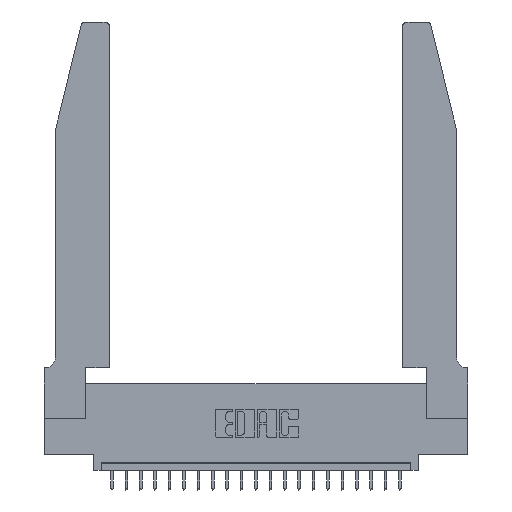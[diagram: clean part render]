
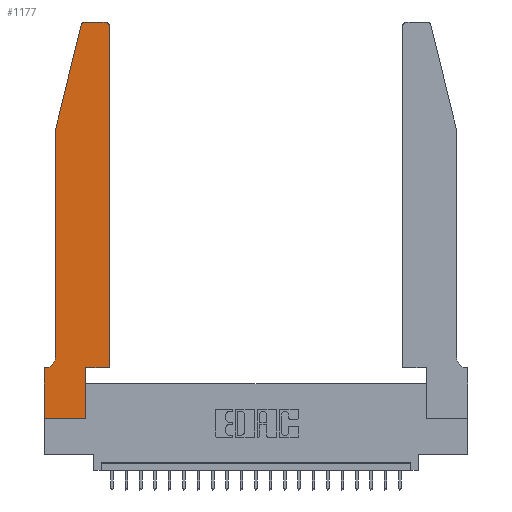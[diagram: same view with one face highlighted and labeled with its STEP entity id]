
A CAD part, top view. The second image highlights one B-rep face of the part: STEP entity #1177.
In plain terms, the highlighted planar face has unit normal (0, 0, 1).
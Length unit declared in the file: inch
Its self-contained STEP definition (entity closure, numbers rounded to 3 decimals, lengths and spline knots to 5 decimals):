
#88 = EDGE_CURVE ( 'NONE', #14024, #15743, #11137, .T. ) ;
#162 = EDGE_CURVE ( 'NONE', #15743, #178, #12578, .T. ) ;
#178 = VERTEX_POINT ( 'NONE', #19952 ) ;
#201 = CARTESIAN_POINT ( 'NONE',  ( 0.2865, 0., 0.37 ) ) ;
#208 = CARTESIAN_POINT ( 'NONE',  ( 0., 0., 0.37 ) ) ;
#233 = VECTOR ( 'NONE', #21987, 39.37008 ) ;
#817 = VECTOR ( 'NONE', #3164, 39.37008 ) ;
#978 = AXIS2_PLACEMENT_3D ( 'NONE', #20829, #2911, #8071 ) ;
#1104 = LINE ( 'NONE', #1340, #17027 ) ;
#1177 = ADVANCED_FACE ( 'NONE', ( #19053 ), #10132, .T. ) ;
#1340 = CARTESIAN_POINT ( 'NONE',  ( 0., 0., 0.37 ) ) ;
#1883 = AXIS2_PLACEMENT_3D ( 'NONE', #6536, #22532, #6172 ) ;
#2139 = ORIENTED_EDGE ( 'NONE', *, *, #17794, .T. ) ;
#2397 = CARTESIAN_POINT ( 'NONE',  ( 0.284, 2.75, 0.37 ) ) ;
#2544 = DIRECTION ( 'NONE',  ( 1., 0., 0. ) ) ;
#2810 = CARTESIAN_POINT ( 'NONE',  ( 0.0755, 0.35, 0.37 ) ) ;
#2911 = DIRECTION ( 'NONE',  ( 0., 0., 1. ) ) ;
#2994 = DIRECTION ( 'NONE',  ( 0., -1., 0. ) ) ;
#3002 = DIRECTION ( 'NONE',  ( 0., 0., 1. ) ) ;
#3164 = DIRECTION ( 'NONE',  ( -1., 0., 0. ) ) ;
#3279 = ORIENTED_EDGE ( 'NONE', *, *, #21808, .T. ) ;
#3718 = ORIENTED_EDGE ( 'NONE', *, *, #12298, .T. ) ;
#3720 = ORIENTED_EDGE ( 'NONE', *, *, #88, .T. ) ;
#3785 = CARTESIAN_POINT ( 'NONE',  ( 0., 0.35, 0.37 ) ) ;
#3889 = VERTEX_POINT ( 'NONE', #208 ) ;
#4787 = VERTEX_POINT ( 'NONE', #6211 ) ;
#4860 = LINE ( 'NONE', #15916, #21438 ) ;
#5354 = ORIENTED_EDGE ( 'NONE', *, *, #162, .T. ) ;
#5496 = VERTEX_POINT ( 'NONE', #12077 ) ;
#6172 = DIRECTION ( 'NONE',  ( 1., 0., 0. ) ) ;
#6211 = CARTESIAN_POINT ( 'NONE',  ( 0.0755, 0.42, 0.37 ) ) ;
#6536 = CARTESIAN_POINT ( 'NONE',  ( 0.284, 2.72, 0.37 ) ) ;
#7305 = ORIENTED_EDGE ( 'NONE', *, *, #10333, .T. ) ;
#7371 = CARTESIAN_POINT ( 'NONE',  ( 0.2865, 0.35, 0.37 ) ) ;
#7953 = EDGE_CURVE ( 'NONE', #22716, #3889, #1104, .T. ) ;
#7985 = VERTEX_POINT ( 'NONE', #15449 ) ;
#8048 = LINE ( 'NONE', #19032, #16364 ) ;
#8071 = DIRECTION ( 'NONE',  ( 1., 0., 0. ) ) ;
#8715 = DIRECTION ( 'NONE',  ( 0., 0., -1. ) ) ;
#9107 = DIRECTION ( 'NONE',  ( 0., 1., 0. ) ) ;
#10132 = PLANE ( 'NONE',  #978 ) ;
#10333 = EDGE_CURVE ( 'NONE', #22520, #19962, #23164, .T. ) ;
#10337 = CARTESIAN_POINT ( 'NONE',  ( 0.4205, 2.72, 0.37 ) ) ;
#11137 = LINE ( 'NONE', #7371, #13256 ) ;
#11561 = DIRECTION ( 'NONE',  ( 1., 0., 0. ) ) ;
#11953 = LINE ( 'NONE', #2810, #817 ) ;
#12077 = CARTESIAN_POINT ( 'NONE',  ( 0.0755, 2., 0.37 ) ) ;
#12244 = CIRCLE ( 'NONE', #1883, 0.03 ) ;
#12298 = EDGE_CURVE ( 'NONE', #7985, #5496, #8048, .T. ) ;
#12326 = CARTESIAN_POINT ( 'NONE',  ( 0.0055, 0.42, 0.37 ) ) ;
#12578 = LINE ( 'NONE', #12822, #233 ) ;
#12766 = VERTEX_POINT ( 'NONE', #16245 ) ;
#12822 = CARTESIAN_POINT ( 'NONE',  ( 0.4505, 0.35, 0.37 ) ) ;
#13021 = AXIS2_PLACEMENT_3D ( 'NONE', #10337, #3002, #2544 ) ;
#13195 = VERTEX_POINT ( 'NONE', #17960 ) ;
#13256 = VECTOR ( 'NONE', #9107, 39.37008 ) ;
#13408 = VECTOR ( 'NONE', #21277, 39.37008 ) ;
#13709 = VECTOR ( 'NONE', #14155, 39.37008 ) ;
#14024 = VERTEX_POINT ( 'NONE', #201 ) ;
#14025 = CARTESIAN_POINT ( 'NONE',  ( 0.0755, 2., 0.37 ) ) ;
#14155 = DIRECTION ( 'NONE',  ( -1., 0., 0. ) ) ;
#14206 = CIRCLE ( 'NONE', #21790, 0.07 ) ;
#14281 = CARTESIAN_POINT ( 'NONE',  ( 0.2605, 2.75, 0.37 ) ) ;
#15152 = LINE ( 'NONE', #20342, #22151 ) ;
#15169 = ORIENTED_EDGE ( 'NONE', *, *, #15344, .T. ) ;
#15172 = EDGE_CURVE ( 'NONE', #5496, #4787, #23040, .T. ) ;
#15261 = EDGE_CURVE ( 'NONE', #19962, #7985, #12244, .T. ) ;
#15319 = CIRCLE ( 'NONE', #13021, 0.03 ) ;
#15344 = EDGE_CURVE ( 'NONE', #3889, #14024, #15152, .T. ) ;
#15449 = CARTESIAN_POINT ( 'NONE',  ( 0.25487, 2.72718, 0.37 ) ) ;
#15743 = VERTEX_POINT ( 'NONE', #18087 ) ;
#15916 = CARTESIAN_POINT ( 'NONE',  ( 0.4505, 0.35, 0.37 ) ) ;
#16024 = DIRECTION ( 'NONE',  ( 0., 1., 0. ) ) ;
#16245 = CARTESIAN_POINT ( 'NONE',  ( 0.0055, 0.35, 0.37 ) ) ;
#16247 = ORIENTED_EDGE ( 'NONE', *, *, #15261, .T. ) ;
#16364 = VECTOR ( 'NONE', #19272, 39.37008 ) ;
#16979 = EDGE_CURVE ( 'NONE', #12766, #22716, #11953, .T. ) ;
#17027 = VECTOR ( 'NONE', #2994, 39.37008 ) ;
#17794 = EDGE_CURVE ( 'NONE', #178, #13195, #4860, .T. ) ;
#17960 = CARTESIAN_POINT ( 'NONE',  ( 0.4505, 2.72, 0.37 ) ) ;
#18087 = CARTESIAN_POINT ( 'NONE',  ( 0.2865, 0.35, 0.37 ) ) ;
#18716 = ORIENTED_EDGE ( 'NONE', *, *, #16979, .T. ) ;
#19032 = CARTESIAN_POINT ( 'NONE',  ( 0.0755, 2., 0.37 ) ) ;
#19053 = FACE_OUTER_BOUND ( 'NONE', #19124, .T. ) ;
#19124 = EDGE_LOOP ( 'NONE', ( #7305, #16247, #3718, #22018, #19297, #18716, #23192, #15169, #3720, #5354, #2139, #3279 ) ) ;
#19272 = DIRECTION ( 'NONE',  ( -0.239, -0.971, 0. ) ) ;
#19297 = ORIENTED_EDGE ( 'NONE', *, *, #22624, .T. ) ;
#19800 = DIRECTION ( 'NONE',  ( -1., 0., 0. ) ) ;
#19952 = CARTESIAN_POINT ( 'NONE',  ( 0.4505, 0.35, 0.37 ) ) ;
#19962 = VERTEX_POINT ( 'NONE', #2397 ) ;
#20342 = CARTESIAN_POINT ( 'NONE',  ( 0., 0., 0.37 ) ) ;
#20829 = CARTESIAN_POINT ( 'NONE',  ( 0., 0.35, 0.37 ) ) ;
#21277 = DIRECTION ( 'NONE',  ( 0., -1., 0. ) ) ;
#21438 = VECTOR ( 'NONE', #16024, 39.37008 ) ;
#21790 = AXIS2_PLACEMENT_3D ( 'NONE', #12326, #8715, #19800 ) ;
#21808 = EDGE_CURVE ( 'NONE', #13195, #22520, #15319, .T. ) ;
#21987 = DIRECTION ( 'NONE',  ( 1., 0., 0. ) ) ;
#22018 = ORIENTED_EDGE ( 'NONE', *, *, #15172, .T. ) ;
#22151 = VECTOR ( 'NONE', #11561, 39.37008 ) ;
#22520 = VERTEX_POINT ( 'NONE', #22668 ) ;
#22532 = DIRECTION ( 'NONE',  ( 0., 0., 1. ) ) ;
#22624 = EDGE_CURVE ( 'NONE', #4787, #12766, #14206, .T. ) ;
#22668 = CARTESIAN_POINT ( 'NONE',  ( 0.4205, 2.75, 0.37 ) ) ;
#22716 = VERTEX_POINT ( 'NONE', #3785 ) ;
#23040 = LINE ( 'NONE', #14025, #13408 ) ;
#23164 = LINE ( 'NONE', #14281, #13709 ) ;
#23192 = ORIENTED_EDGE ( 'NONE', *, *, #7953, .T. ) ;
